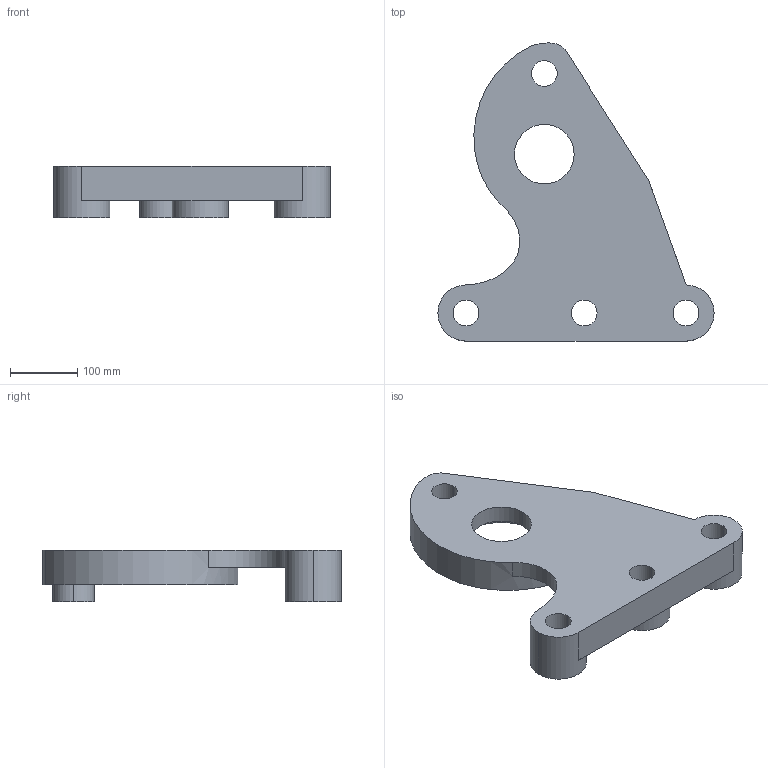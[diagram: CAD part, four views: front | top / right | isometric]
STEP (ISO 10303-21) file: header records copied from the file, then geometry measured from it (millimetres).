
FILE_DESCRIPTION (( 'STEP AP214' ), '1' );
FILE_NAME ('Plate_1.STEP', '2014-02-05T15:25:30', ( 'elpi' ), ( '' ), 'SwSTEP 2.0', 'SolidWorks 2013', '' );
FILE_SCHEMA (( 'AUTOMOTIVE_DESIGN' ));
Length unit declared in the file: inch
Products named in the file (1): Plate_1
Bounding box: 410.4 x 443.01 x 76.2 mm (x, y, z)
Volume: 4320646 mm3; surface area: 359075.5 mm2
Topology: 1 solids, 1 shells, 40 faces, 106 edges, 70 vertices
Faces by surface type: cylinder 21, plane 16, bspline 3
Entity records: 1335 total; most frequent: CARTESIAN_POINT 255, DIRECTION 221, ORIENTED_EDGE 212, EDGE_CURVE 106, AXIS2_PLACEMENT_3D 84, VERTEX_POINT 70, LINE 53, VECTOR 53
